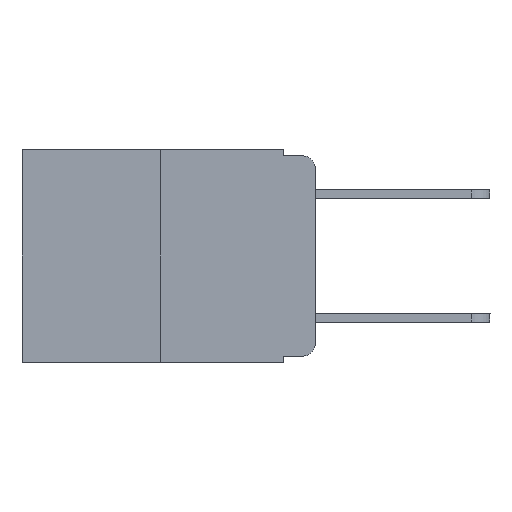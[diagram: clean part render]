
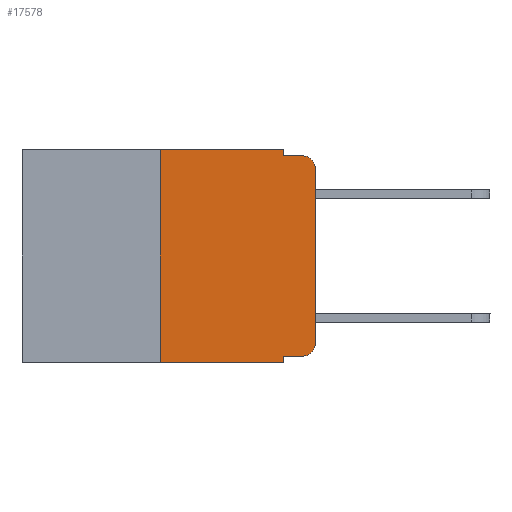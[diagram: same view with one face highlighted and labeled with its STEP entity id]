
A CAD part, left-side view. The second image highlights one B-rep face of the part: STEP entity #17578.
In plain terms, the highlighted planar face has unit normal (-1, 0, 0).
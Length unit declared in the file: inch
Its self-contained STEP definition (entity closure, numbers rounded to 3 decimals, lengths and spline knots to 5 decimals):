
#57 = VERTEX_POINT ( 'NONE', #6937 ) ;
#137 = VECTOR ( 'NONE', #21310, 39.37008 ) ;
#185 = VECTOR ( 'NONE', #9127, 39.37008 ) ;
#624 = CIRCLE ( 'NONE', #1463, 0.02 ) ;
#1435 = CARTESIAN_POINT ( 'NONE',  ( 0., 0., -0.313 ) ) ;
#1463 = AXIS2_PLACEMENT_3D ( 'NONE', #15148, #5343, #19331 ) ;
#1827 = DIRECTION ( 'NONE',  ( 0., 0., -1. ) ) ;
#2167 = CARTESIAN_POINT ( 'NONE',  ( 0., 0.25, 0. ) ) ;
#2229 = VERTEX_POINT ( 'NONE', #18276 ) ;
#2309 = EDGE_CURVE ( 'NONE', #4473, #19933, #624, .T. ) ;
#2433 = LINE ( 'NONE', #19302, #17735 ) ;
#2988 = ORIENTED_EDGE ( 'NONE', *, *, #21233, .F. ) ;
#3648 = ORIENTED_EDGE ( 'NONE', *, *, #9302, .F. ) ;
#3714 = DIRECTION ( 'NONE',  ( 0., 0., -1. ) ) ;
#4097 = CARTESIAN_POINT ( 'NONE',  ( 0., 0.02, -0.03 ) ) ;
#4190 = DIRECTION ( 'NONE',  ( 0., 0., 1. ) ) ;
#4473 = VERTEX_POINT ( 'NONE', #18479 ) ;
#4944 = EDGE_CURVE ( 'NONE', #5922, #25219, #23357, .T. ) ;
#5343 = DIRECTION ( 'NONE',  ( -1., 0., 0. ) ) ;
#5430 = LINE ( 'NONE', #11020, #18232 ) ;
#5922 = VERTEX_POINT ( 'NONE', #12569 ) ;
#6267 = ORIENTED_EDGE ( 'NONE', *, *, #10088, .F. ) ;
#6288 = LINE ( 'NONE', #19509, #16591 ) ;
#6562 = ORIENTED_EDGE ( 'NONE', *, *, #2309, .T. ) ;
#6937 = CARTESIAN_POINT ( 'NONE',  ( 0., 0.051, 0. ) ) ;
#7124 = DIRECTION ( 'NONE',  ( 1., 0., 0. ) ) ;
#7612 = CARTESIAN_POINT ( 'NONE',  ( 0., 0.051, -0.01 ) ) ;
#7655 = VECTOR ( 'NONE', #11048, 39.37008 ) ;
#7774 = CARTESIAN_POINT ( 'NONE',  ( 0., 0.051, -0.343 ) ) ;
#8395 = EDGE_CURVE ( 'NONE', #19933, #5922, #2433, .T. ) ;
#9127 = DIRECTION ( 'NONE',  ( 0., 0., -1. ) ) ;
#9302 = EDGE_CURVE ( 'NONE', #57, #18319, #11427, .T. ) ;
#10088 = EDGE_CURVE ( 'NONE', #15068, #10233, #15775, .T. ) ;
#10220 = ORIENTED_EDGE ( 'NONE', *, *, #8395, .T. ) ;
#10233 = VERTEX_POINT ( 'NONE', #7774 ) ;
#11020 = CARTESIAN_POINT ( 'NONE',  ( 0., 0.051, -0.01 ) ) ;
#11048 = DIRECTION ( 'NONE',  ( 0., -1., 0. ) ) ;
#11427 = LINE ( 'NONE', #15262, #185 ) ;
#11559 = LINE ( 'NONE', #2167, #24648 ) ;
#12284 = EDGE_CURVE ( 'NONE', #18319, #25219, #5430, .T. ) ;
#12569 = CARTESIAN_POINT ( 'NONE',  ( 0., 0., -0.03 ) ) ;
#12895 = EDGE_LOOP ( 'NONE', ( #10220, #13458, #14461, #3648, #25672, #2988, #13254, #6267, #18599, #6562 ) ) ;
#13162 = PLANE ( 'NONE',  #14730 ) ;
#13254 = ORIENTED_EDGE ( 'NONE', *, *, #15106, .T. ) ;
#13255 = DIRECTION ( 'NONE',  ( 0., -1., 0. ) ) ;
#13458 = ORIENTED_EDGE ( 'NONE', *, *, #4944, .T. ) ;
#14461 = ORIENTED_EDGE ( 'NONE', *, *, #12284, .F. ) ;
#14730 = AXIS2_PLACEMENT_3D ( 'NONE', #19103, #7124, #14747 ) ;
#14747 = DIRECTION ( 'NONE',  ( 0., 0., -1. ) ) ;
#14844 = VECTOR ( 'NONE', #3714, 39.37008 ) ;
#15068 = VERTEX_POINT ( 'NONE', #22486 ) ;
#15106 = EDGE_CURVE ( 'NONE', #2229, #10233, #23589, .T. ) ;
#15148 = CARTESIAN_POINT ( 'NONE',  ( 0., 0.02, -0.313 ) ) ;
#15242 = CARTESIAN_POINT ( 'NONE',  ( 0., 0.25, 0. ) ) ;
#15262 = CARTESIAN_POINT ( 'NONE',  ( 0., 0.051, 0. ) ) ;
#15775 = LINE ( 'NONE', #19593, #14844 ) ;
#16141 = EDGE_CURVE ( 'NONE', #15068, #4473, #6288, .T. ) ;
#16591 = VECTOR ( 'NONE', #17485, 39.37008 ) ;
#17030 = FACE_OUTER_BOUND ( 'NONE', #12895, .T. ) ;
#17485 = DIRECTION ( 'NONE',  ( 0., -1., 0. ) ) ;
#17578 = ADVANCED_FACE ( 'NONE', ( #17030 ), #13162, .F. ) ;
#17735 = VECTOR ( 'NONE', #17802, 39.37008 ) ;
#17797 = DIRECTION ( 'NONE',  ( -1., 0., 0. ) ) ;
#17802 = DIRECTION ( 'NONE',  ( 0., 0., 1. ) ) ;
#18232 = VECTOR ( 'NONE', #13255, 39.37008 ) ;
#18276 = CARTESIAN_POINT ( 'NONE',  ( 0., 0.25, -0.343 ) ) ;
#18319 = VERTEX_POINT ( 'NONE', #7612 ) ;
#18479 = CARTESIAN_POINT ( 'NONE',  ( 0., 0.02, -0.333 ) ) ;
#18599 = ORIENTED_EDGE ( 'NONE', *, *, #16141, .T. ) ;
#18778 = EDGE_CURVE ( 'NONE', #25808, #57, #20710, .T. ) ;
#18903 = AXIS2_PLACEMENT_3D ( 'NONE', #4097, #17797, #1827 ) ;
#18980 = CARTESIAN_POINT ( 'NONE',  ( 0., 0.473, -0.343 ) ) ;
#19103 = CARTESIAN_POINT ( 'NONE',  ( 0., 0.473, 0. ) ) ;
#19302 = CARTESIAN_POINT ( 'NONE',  ( 0., 0., 0. ) ) ;
#19331 = DIRECTION ( 'NONE',  ( 0., 0., -1. ) ) ;
#19509 = CARTESIAN_POINT ( 'NONE',  ( 0., 0.051, -0.333 ) ) ;
#19593 = CARTESIAN_POINT ( 'NONE',  ( 0., 0.051, 0. ) ) ;
#19933 = VERTEX_POINT ( 'NONE', #1435 ) ;
#20710 = LINE ( 'NONE', #24882, #137 ) ;
#21233 = EDGE_CURVE ( 'NONE', #2229, #25808, #11559, .T. ) ;
#21310 = DIRECTION ( 'NONE',  ( 0., -1., 0. ) ) ;
#22486 = CARTESIAN_POINT ( 'NONE',  ( 0., 0.051, -0.333 ) ) ;
#23357 = CIRCLE ( 'NONE', #18903, 0.02 ) ;
#23589 = LINE ( 'NONE', #18980, #7655 ) ;
#24648 = VECTOR ( 'NONE', #4190, 39.37008 ) ;
#24882 = CARTESIAN_POINT ( 'NONE',  ( 0., 0.473, 0. ) ) ;
#24919 = CARTESIAN_POINT ( 'NONE',  ( 0., 0.02, -0.01 ) ) ;
#25219 = VERTEX_POINT ( 'NONE', #24919 ) ;
#25672 = ORIENTED_EDGE ( 'NONE', *, *, #18778, .F. ) ;
#25808 = VERTEX_POINT ( 'NONE', #15242 ) ;
